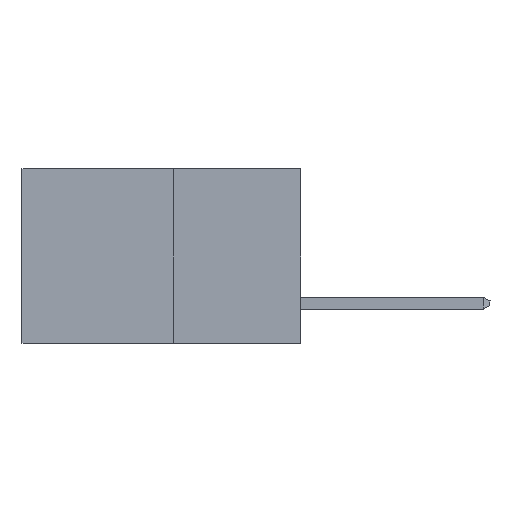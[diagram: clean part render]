
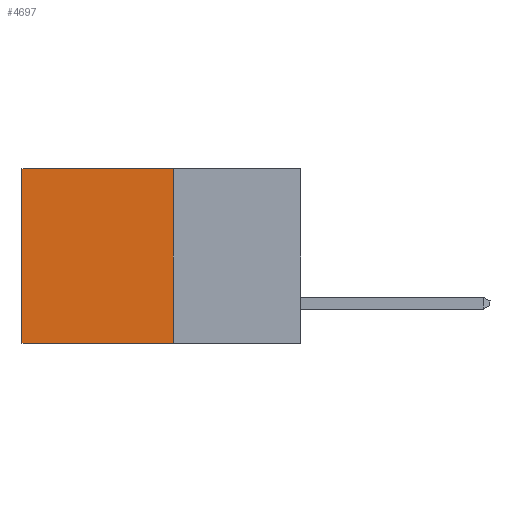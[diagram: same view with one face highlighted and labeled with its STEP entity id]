
A CAD part, left-side view. The second image highlights one B-rep face of the part: STEP entity #4697.
In plain terms, the highlighted planar face has unit normal (-1, 0, 0).
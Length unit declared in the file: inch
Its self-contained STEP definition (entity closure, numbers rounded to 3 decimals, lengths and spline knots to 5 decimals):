
#127 = VECTOR ( 'NONE', #4262, 39.37008 ) ;
#175 = VERTEX_POINT ( 'NONE', #5028 ) ;
#367 = LINE ( 'NONE', #4251, #127 ) ;
#508 = PLANE ( 'NONE',  #4950 ) ;
#643 = FACE_OUTER_BOUND ( 'NONE', #6523, .T. ) ;
#658 = CARTESIAN_POINT ( 'NONE',  ( 0.277, 0.59, -0.37 ) ) ;
#1020 = LINE ( 'NONE', #5077, #6603 ) ;
#1201 = CARTESIAN_POINT ( 'NONE',  ( 0.277, 0.27, -0.37 ) ) ;
#1390 = EDGE_CURVE ( 'NONE', #175, #5153, #1020, .T. ) ;
#1403 = VERTEX_POINT ( 'NONE', #5898 ) ;
#1497 = ORIENTED_EDGE ( 'NONE', *, *, #2532, .T. ) ;
#1518 = DIRECTION ( 'NONE',  ( 1., 0., 0. ) ) ;
#1794 = DIRECTION ( 'NONE',  ( 0., 0., -1. ) ) ;
#2103 = VERTEX_POINT ( 'NONE', #3273 ) ;
#2185 = ORIENTED_EDGE ( 'NONE', *, *, #9102, .F. ) ;
#2396 = VECTOR ( 'NONE', #4718, 39.37008 ) ;
#2532 = EDGE_CURVE ( 'NONE', #1403, #5153, #4592, .T. ) ;
#3001 = ORIENTED_EDGE ( 'NONE', *, *, #1390, .F. ) ;
#3136 = VECTOR ( 'NONE', #8460, 39.37008 ) ;
#3273 = CARTESIAN_POINT ( 'NONE',  ( 0.277, 0.27, 0. ) ) ;
#4251 = CARTESIAN_POINT ( 'NONE',  ( 0.277, 0.27, 0. ) ) ;
#4262 = DIRECTION ( 'NONE',  ( 0., 1., 0. ) ) ;
#4592 = LINE ( 'NONE', #658, #2396 ) ;
#4697 = ADVANCED_FACE ( 'NONE', ( #643 ), #508, .F. ) ;
#4718 = DIRECTION ( 'NONE',  ( 0., 0., -1. ) ) ;
#4950 = AXIS2_PLACEMENT_3D ( 'NONE', #1201, #1518, #1794 ) ;
#5028 = CARTESIAN_POINT ( 'NONE',  ( 0.277, 0.27, -0.37 ) ) ;
#5077 = CARTESIAN_POINT ( 'NONE',  ( 0.277, 0.27, -0.37 ) ) ;
#5153 = VERTEX_POINT ( 'NONE', #8626 ) ;
#5898 = CARTESIAN_POINT ( 'NONE',  ( 0.277, 0.59, 0. ) ) ;
#6484 = EDGE_CURVE ( 'NONE', #2103, #1403, #367, .T. ) ;
#6523 = EDGE_LOOP ( 'NONE', ( #1497, #3001, #2185, #6783 ) ) ;
#6603 = VECTOR ( 'NONE', #8951, 39.37008 ) ;
#6783 = ORIENTED_EDGE ( 'NONE', *, *, #6484, .T. ) ;
#7735 = CARTESIAN_POINT ( 'NONE',  ( 0.277, 0.27, -0.37 ) ) ;
#8460 = DIRECTION ( 'NONE',  ( 0., 0., -1. ) ) ;
#8626 = CARTESIAN_POINT ( 'NONE',  ( 0.277, 0.59, -0.37 ) ) ;
#8866 = LINE ( 'NONE', #7735, #3136 ) ;
#8951 = DIRECTION ( 'NONE',  ( 0., 1., 0. ) ) ;
#9102 = EDGE_CURVE ( 'NONE', #2103, #175, #8866, .T. ) ;
